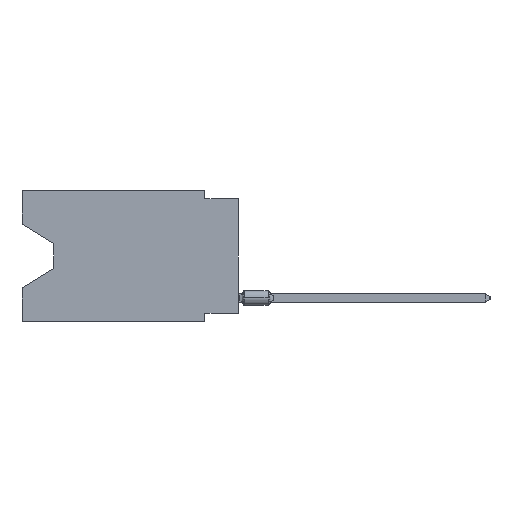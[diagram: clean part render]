
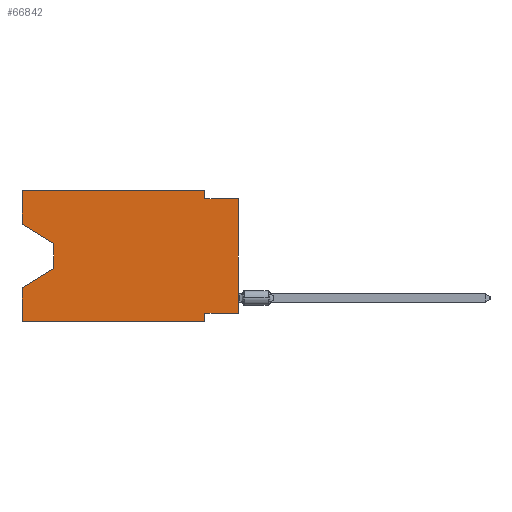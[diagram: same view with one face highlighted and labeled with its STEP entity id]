
A CAD part, left-side view. The second image highlights one B-rep face of the part: STEP entity #66842.
In plain terms, the highlighted planar face has unit normal (-1, 0, 0).
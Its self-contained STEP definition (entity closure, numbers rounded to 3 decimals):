
#191 = DIRECTION ( 'NONE',  ( 0., 0., -1. ) ) ;
#3400 = EDGE_CURVE ( 'NONE', #34676, #61544, #21989, .T. ) ;
#5217 = VERTEX_POINT ( 'NONE', #83474 ) ;
#5783 = VECTOR ( 'NONE', #17924, 1000. ) ;
#7657 = CARTESIAN_POINT ( 'NONE',  ( 0., 2.54, 0. ) ) ;
#8215 = EDGE_LOOP ( 'NONE', ( #10367, #74271, #75847, #60808, #32073, #83063, #72740, #18674, #50360, #15558, #62180, #8351 ) ) ;
#8351 = ORIENTED_EDGE ( 'NONE', *, *, #48991, .F. ) ;
#8406 = CARTESIAN_POINT ( 'NONE',  ( 0., 0., -9.271 ) ) ;
#9203 = EDGE_CURVE ( 'NONE', #34676, #30346, #50683, .T. ) ;
#10208 = CARTESIAN_POINT ( 'NONE',  ( 0., 16.383, -7.36 ) ) ;
#10297 = VERTEX_POINT ( 'NONE', #10208 ) ;
#10367 = ORIENTED_EDGE ( 'NONE', *, *, #21562, .T. ) ;
#10798 = VERTEX_POINT ( 'NONE', #20102 ) ;
#11974 = CARTESIAN_POINT ( 'NONE',  ( 0., 16.383, 0. ) ) ;
#13864 = DIRECTION ( 'NONE',  ( 0., 0., -1. ) ) ;
#14287 = CARTESIAN_POINT ( 'NONE',  ( 0., 16.383, -2.546 ) ) ;
#15558 = ORIENTED_EDGE ( 'NONE', *, *, #43892, .F. ) ;
#17501 = DIRECTION ( 'NONE',  ( 0., -1., 0. ) ) ;
#17924 = DIRECTION ( 'NONE',  ( 0., 0., 1. ) ) ;
#18674 = ORIENTED_EDGE ( 'NONE', *, *, #9203, .T. ) ;
#20102 = CARTESIAN_POINT ( 'NONE',  ( 0., 16.383, 0. ) ) ;
#21562 = EDGE_CURVE ( 'NONE', #71903, #61452, #28155, .T. ) ;
#21989 = LINE ( 'NONE', #8406, #22225 ) ;
#22203 = DIRECTION ( 'NONE',  ( 0., -1., 0. ) ) ;
#22225 = VECTOR ( 'NONE', #60653, 1000. ) ;
#22611 = LINE ( 'NONE', #37461, #60147 ) ;
#22979 = FACE_OUTER_BOUND ( 'NONE', #8215, .T. ) ;
#23397 = DIRECTION ( 'NONE',  ( 1., 0., 0. ) ) ;
#23433 = CARTESIAN_POINT ( 'NONE',  ( 0., 16.383, -9.906 ) ) ;
#28155 = LINE ( 'NONE', #61284, #45986 ) ;
#29402 = CARTESIAN_POINT ( 'NONE',  ( 0., 16.383, -9.906 ) ) ;
#29767 = PLANE ( 'NONE',  #49917 ) ;
#30346 = VERTEX_POINT ( 'NONE', #47135 ) ;
#31138 = CARTESIAN_POINT ( 'NONE',  ( 0., 2.54, -9.271 ) ) ;
#31697 = CARTESIAN_POINT ( 'NONE',  ( 0., 2.54, -0.635 ) ) ;
#32073 = ORIENTED_EDGE ( 'NONE', *, *, #45397, .T. ) ;
#32313 = DIRECTION ( 'NONE',  ( 0., 0., -1. ) ) ;
#32939 = CARTESIAN_POINT ( 'NONE',  ( 0., 2.54, 0. ) ) ;
#33981 = LINE ( 'NONE', #7657, #76092 ) ;
#34676 = VERTEX_POINT ( 'NONE', #35440 ) ;
#35440 = CARTESIAN_POINT ( 'NONE',  ( 0., 0., -9.271 ) ) ;
#37461 = CARTESIAN_POINT ( 'NONE',  ( 0., 16.383, 0. ) ) ;
#37656 = DIRECTION ( 'NONE',  ( 0., 0.855, -0.519 ) ) ;
#37950 = CARTESIAN_POINT ( 'NONE',  ( 0., 0., 0. ) ) ;
#39221 = CARTESIAN_POINT ( 'NONE',  ( 0., 0., -0.635 ) ) ;
#43672 = CARTESIAN_POINT ( 'NONE',  ( 0., 2.54, -9.906 ) ) ;
#43892 = EDGE_CURVE ( 'NONE', #75544, #66246, #33981, .T. ) ;
#44265 = LINE ( 'NONE', #11974, #5783 ) ;
#45397 = EDGE_CURVE ( 'NONE', #65694, #66137, #75718, .T. ) ;
#45439 = EDGE_CURVE ( 'NONE', #10798, #75544, #22611, .T. ) ;
#45986 = VECTOR ( 'NONE', #54063, 1000. ) ;
#46424 = VECTOR ( 'NONE', #37656, 1000. ) ;
#46716 = VECTOR ( 'NONE', #49408, 1000. ) ;
#47135 = CARTESIAN_POINT ( 'NONE',  ( 0., 0., -0.635 ) ) ;
#48991 = EDGE_CURVE ( 'NONE', #71903, #10798, #44265, .T. ) ;
#49408 = DIRECTION ( 'NONE',  ( 0., 0., 1. ) ) ;
#49917 = AXIS2_PLACEMENT_3D ( 'NONE', #55681, #23397, #61476 ) ;
#50360 = ORIENTED_EDGE ( 'NONE', *, *, #53752, .F. ) ;
#50630 = VECTOR ( 'NONE', #17501, 1000. ) ;
#50683 = LINE ( 'NONE', #37950, #60355 ) ;
#50936 = EDGE_CURVE ( 'NONE', #61452, #5217, #79725, .T. ) ;
#51970 = LINE ( 'NONE', #39221, #52060 ) ;
#52060 = VECTOR ( 'NONE', #22203, 1000. ) ;
#53752 = EDGE_CURVE ( 'NONE', #66246, #30346, #51970, .T. ) ;
#54063 = DIRECTION ( 'NONE',  ( 0., -0.855, -0.519 ) ) ;
#55379 = CARTESIAN_POINT ( 'NONE',  ( 0., 13.97, -4.013 ) ) ;
#55681 = CARTESIAN_POINT ( 'NONE',  ( 0., 16.383, 0. ) ) ;
#56203 = LINE ( 'NONE', #68966, #46716 ) ;
#58389 = LINE ( 'NONE', #43672, #61120 ) ;
#60147 = VECTOR ( 'NONE', #62118, 1000. ) ;
#60179 = CARTESIAN_POINT ( 'NONE',  ( 0., 13.97, -4.013 ) ) ;
#60304 = EDGE_CURVE ( 'NONE', #65694, #10297, #56203, .T. ) ;
#60355 = VECTOR ( 'NONE', #63864, 1000. ) ;
#60653 = DIRECTION ( 'NONE',  ( 0., 1., 0. ) ) ;
#60808 = ORIENTED_EDGE ( 'NONE', *, *, #60304, .F. ) ;
#61120 = VECTOR ( 'NONE', #191, 1000. ) ;
#61284 = CARTESIAN_POINT ( 'NONE',  ( 0., 16.383, -2.546 ) ) ;
#61452 = VERTEX_POINT ( 'NONE', #55379 ) ;
#61476 = DIRECTION ( 'NONE',  ( 0., 0., -1. ) ) ;
#61544 = VERTEX_POINT ( 'NONE', #31138 ) ;
#62118 = DIRECTION ( 'NONE',  ( 0., -1., 0. ) ) ;
#62180 = ORIENTED_EDGE ( 'NONE', *, *, #45439, .F. ) ;
#63864 = DIRECTION ( 'NONE',  ( 0., 0., 1. ) ) ;
#63993 = CARTESIAN_POINT ( 'NONE',  ( 0., 13.97, -5.893 ) ) ;
#65694 = VERTEX_POINT ( 'NONE', #23433 ) ;
#66137 = VERTEX_POINT ( 'NONE', #81861 ) ;
#66246 = VERTEX_POINT ( 'NONE', #31697 ) ;
#66842 = ADVANCED_FACE ( 'NONE', ( #22979 ), #29767, .F. ) ;
#68966 = CARTESIAN_POINT ( 'NONE',  ( 0., 16.383, 0. ) ) ;
#71903 = VERTEX_POINT ( 'NONE', #14287 ) ;
#72740 = ORIENTED_EDGE ( 'NONE', *, *, #3400, .F. ) ;
#74271 = ORIENTED_EDGE ( 'NONE', *, *, #50936, .T. ) ;
#75544 = VERTEX_POINT ( 'NONE', #32939 ) ;
#75718 = LINE ( 'NONE', #29402, #50630 ) ;
#75847 = ORIENTED_EDGE ( 'NONE', *, *, #83697, .T. ) ;
#76092 = VECTOR ( 'NONE', #32313, 1000. ) ;
#76338 = LINE ( 'NONE', #63993, #46424 ) ;
#79284 = VECTOR ( 'NONE', #13864, 1000. ) ;
#79725 = LINE ( 'NONE', #60179, #79284 ) ;
#81437 = EDGE_CURVE ( 'NONE', #61544, #66137, #58389, .T. ) ;
#81861 = CARTESIAN_POINT ( 'NONE',  ( 0., 2.54, -9.906 ) ) ;
#83063 = ORIENTED_EDGE ( 'NONE', *, *, #81437, .F. ) ;
#83474 = CARTESIAN_POINT ( 'NONE',  ( 0., 13.97, -5.893 ) ) ;
#83697 = EDGE_CURVE ( 'NONE', #5217, #10297, #76338, .T. ) ;
